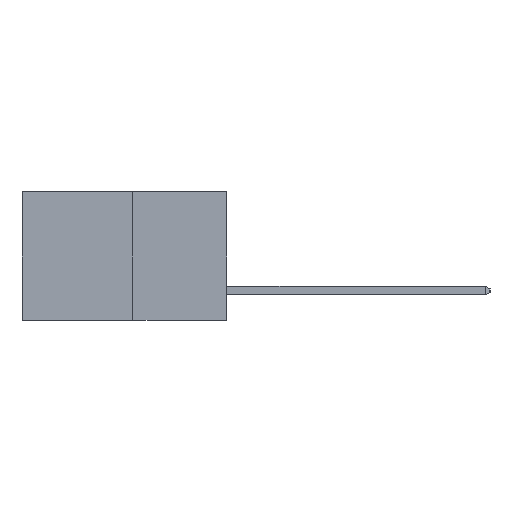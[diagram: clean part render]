
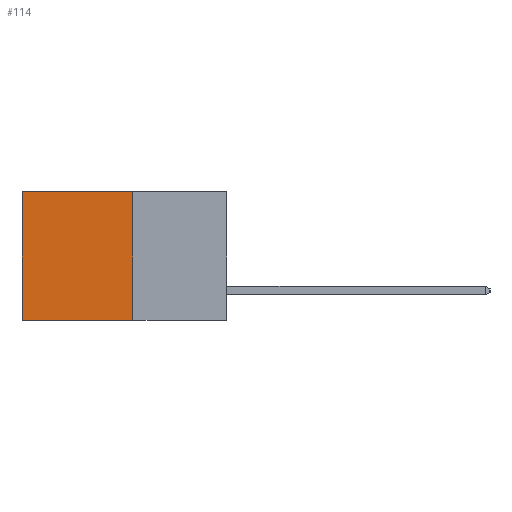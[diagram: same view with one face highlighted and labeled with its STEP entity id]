
A CAD part, left-side view. The second image highlights one B-rep face of the part: STEP entity #114.
In plain terms, the highlighted planar face has unit normal (-1, 0, 0).
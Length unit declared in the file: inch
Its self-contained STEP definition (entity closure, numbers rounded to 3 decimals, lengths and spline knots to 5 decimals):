
#4 = VECTOR ( 'NONE', #6748, 39.37008 ) ;
#114 = ADVANCED_FACE ( 'NONE', ( #8257 ), #7467, .F. ) ;
#744 = EDGE_CURVE ( 'NONE', #5520, #8731, #10661, .T. ) ;
#1017 = LINE ( 'NONE', #13659, #8107 ) ;
#2936 = ORIENTED_EDGE ( 'NONE', *, *, #744, .T. ) ;
#3106 = VECTOR ( 'NONE', #14272, 39.37008 ) ;
#3281 = ORIENTED_EDGE ( 'NONE', *, *, #5668, .F. ) ;
#3395 = ORIENTED_EDGE ( 'NONE', *, *, #4663, .F. ) ;
#3883 = ORIENTED_EDGE ( 'NONE', *, *, #4912, .T. ) ;
#4234 = LINE ( 'NONE', #10357, #4 ) ;
#4293 = CARTESIAN_POINT ( 'NONE',  ( 0.277, 0.27, -0.37 ) ) ;
#4663 = EDGE_CURVE ( 'NONE', #5520, #14526, #4234, .T. ) ;
#4912 = EDGE_CURVE ( 'NONE', #8731, #10987, #1017, .T. ) ;
#5520 = VERTEX_POINT ( 'NONE', #17398 ) ;
#5668 = EDGE_CURVE ( 'NONE', #14526, #10987, #10455, .T. ) ;
#5869 = DIRECTION ( 'NONE',  ( 0., 1., 0. ) ) ;
#6437 = CARTESIAN_POINT ( 'NONE',  ( 0.277, 0.27, -0.37 ) ) ;
#6748 = DIRECTION ( 'NONE',  ( 0., 0., -1. ) ) ;
#6869 = DIRECTION ( 'NONE',  ( 0., 0., -1. ) ) ;
#7467 = PLANE ( 'NONE',  #11194 ) ;
#7934 = DIRECTION ( 'NONE',  ( 1., 0., 0. ) ) ;
#8107 = VECTOR ( 'NONE', #12543, 39.37008 ) ;
#8257 = FACE_OUTER_BOUND ( 'NONE', #11547, .T. ) ;
#8731 = VERTEX_POINT ( 'NONE', #14477 ) ;
#10357 = CARTESIAN_POINT ( 'NONE',  ( 0.277, 0.27, -0.37 ) ) ;
#10455 = LINE ( 'NONE', #4293, #13545 ) ;
#10661 = LINE ( 'NONE', #14190, #3106 ) ;
#10987 = VERTEX_POINT ( 'NONE', #11414 ) ;
#11194 = AXIS2_PLACEMENT_3D ( 'NONE', #6437, #7934, #6869 ) ;
#11414 = CARTESIAN_POINT ( 'NONE',  ( 0.277, 0.59, -0.37 ) ) ;
#11547 = EDGE_LOOP ( 'NONE', ( #3883, #3281, #3395, #2936 ) ) ;
#12543 = DIRECTION ( 'NONE',  ( 0., 0., -1. ) ) ;
#13545 = VECTOR ( 'NONE', #5869, 39.37008 ) ;
#13659 = CARTESIAN_POINT ( 'NONE',  ( 0.277, 0.59, -0.37 ) ) ;
#14190 = CARTESIAN_POINT ( 'NONE',  ( 0.277, 0.27, 0. ) ) ;
#14272 = DIRECTION ( 'NONE',  ( 0., 1., 0. ) ) ;
#14477 = CARTESIAN_POINT ( 'NONE',  ( 0.277, 0.59, 0. ) ) ;
#14506 = CARTESIAN_POINT ( 'NONE',  ( 0.277, 0.27, -0.37 ) ) ;
#14526 = VERTEX_POINT ( 'NONE', #14506 ) ;
#17398 = CARTESIAN_POINT ( 'NONE',  ( 0.277, 0.27, 0. ) ) ;
